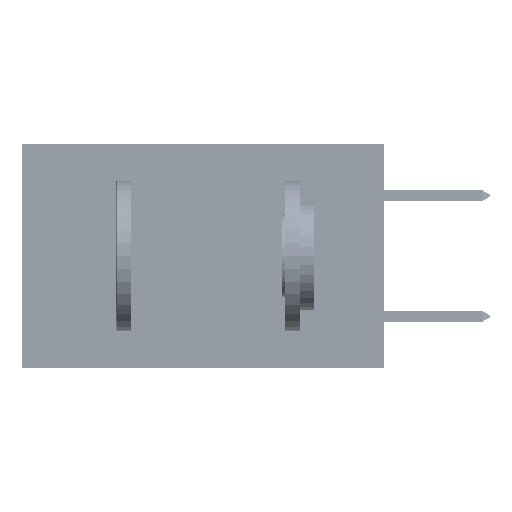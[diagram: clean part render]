
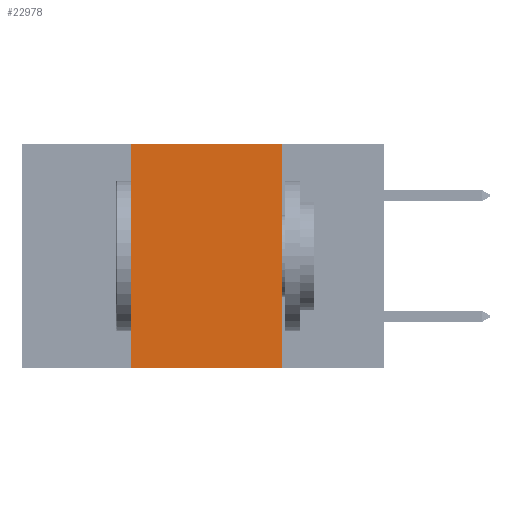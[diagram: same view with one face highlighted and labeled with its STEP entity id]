
A CAD part, left-side view. The second image highlights one B-rep face of the part: STEP entity #22978.
In plain terms, the highlighted planar face has unit normal (-1, 0, 0).
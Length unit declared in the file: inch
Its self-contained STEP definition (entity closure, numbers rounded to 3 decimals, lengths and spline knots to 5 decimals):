
#1113 = PLANE ( 'NONE',  #43245 ) ;
#2327 = DIRECTION ( 'NONE',  ( 0., -1., 0. ) ) ;
#3702 = ORIENTED_EDGE ( 'NONE', *, *, #3888, .T. ) ;
#3888 = EDGE_CURVE ( 'NONE', #17505, #33341, #11745, .T. ) ;
#4695 = DIRECTION ( 'NONE',  ( 1., 0., 0. ) ) ;
#5586 = LINE ( 'NONE', #8662, #32142 ) ;
#7540 = CARTESIAN_POINT ( 'NONE',  ( 0., 0.42, 0. ) ) ;
#8131 = ORIENTED_EDGE ( 'NONE', *, *, #13842, .F. ) ;
#8360 = EDGE_CURVE ( 'NONE', #17505, #26454, #37141, .T. ) ;
#8662 = CARTESIAN_POINT ( 'NONE',  ( 0., 0.6, 0. ) ) ;
#9434 = CARTESIAN_POINT ( 'NONE',  ( 0., 0.6, -0.37 ) ) ;
#11745 = LINE ( 'NONE', #9434, #38242 ) ;
#12365 = LINE ( 'NONE', #44559, #38862 ) ;
#13842 = EDGE_CURVE ( 'NONE', #43683, #33341, #12365, .T. ) ;
#15594 = DIRECTION ( 'NONE',  ( 0., -1., 0. ) ) ;
#16180 = EDGE_LOOP ( 'NONE', ( #8131, #34621, #22185, #3702 ) ) ;
#17343 = CARTESIAN_POINT ( 'NONE',  ( 0., 0.42, 0. ) ) ;
#17505 = VERTEX_POINT ( 'NONE', #27675 ) ;
#19230 = EDGE_CURVE ( 'NONE', #26454, #43683, #5586, .T. ) ;
#22185 = ORIENTED_EDGE ( 'NONE', *, *, #8360, .F. ) ;
#22978 = ADVANCED_FACE ( 'NONE', ( #34895 ), #1113, .F. ) ;
#23883 = DIRECTION ( 'NONE',  ( 0., 0., -1. ) ) ;
#24194 = CARTESIAN_POINT ( 'NONE',  ( 0., 0.17, -0.37 ) ) ;
#26454 = VERTEX_POINT ( 'NONE', #17343 ) ;
#27675 = CARTESIAN_POINT ( 'NONE',  ( 0., 0.42, -0.37 ) ) ;
#27950 = VECTOR ( 'NONE', #31739, 39.37008 ) ;
#28936 = DIRECTION ( 'NONE',  ( 0., 0., -1. ) ) ;
#31739 = DIRECTION ( 'NONE',  ( 0., 0., 1. ) ) ;
#32142 = VECTOR ( 'NONE', #15594, 39.37008 ) ;
#33341 = VERTEX_POINT ( 'NONE', #24194 ) ;
#34621 = ORIENTED_EDGE ( 'NONE', *, *, #19230, .F. ) ;
#34895 = FACE_OUTER_BOUND ( 'NONE', #16180, .T. ) ;
#37141 = LINE ( 'NONE', #7540, #27950 ) ;
#38226 = CARTESIAN_POINT ( 'NONE',  ( 0., 0.17, 0. ) ) ;
#38242 = VECTOR ( 'NONE', #2327, 39.37008 ) ;
#38862 = VECTOR ( 'NONE', #23883, 39.37008 ) ;
#42644 = CARTESIAN_POINT ( 'NONE',  ( 0., 0.6, 0. ) ) ;
#43245 = AXIS2_PLACEMENT_3D ( 'NONE', #42644, #4695, #28936 ) ;
#43683 = VERTEX_POINT ( 'NONE', #38226 ) ;
#44559 = CARTESIAN_POINT ( 'NONE',  ( 0., 0.17, 0. ) ) ;
